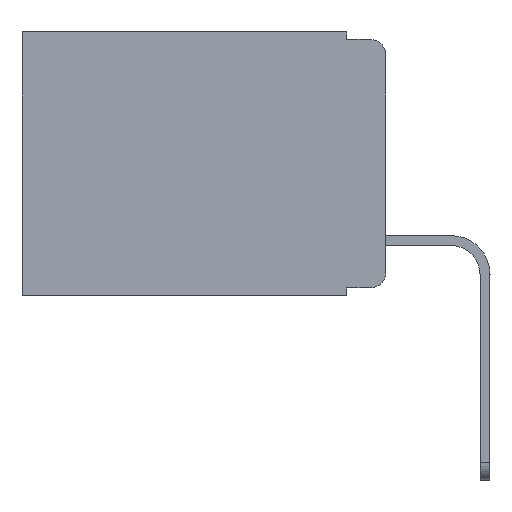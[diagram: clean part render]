
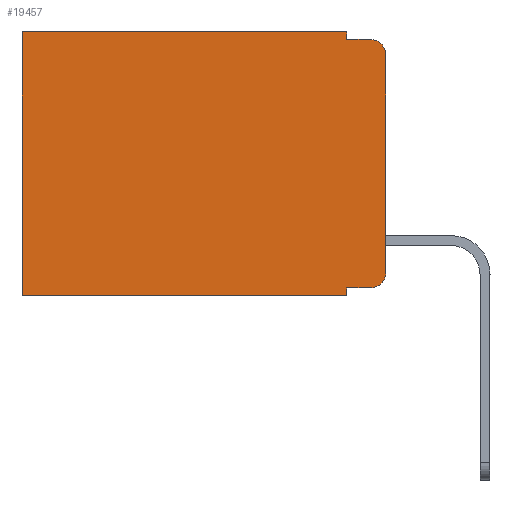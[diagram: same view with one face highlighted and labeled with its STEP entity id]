
A CAD part, left-side view. The second image highlights one B-rep face of the part: STEP entity #19457.
In plain terms, the highlighted planar face has unit normal (-1, 0, 0).
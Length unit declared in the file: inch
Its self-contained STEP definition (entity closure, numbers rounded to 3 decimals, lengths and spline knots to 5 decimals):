
#99 = LINE ( 'NONE', #16720, #21106 ) ;
#116 = VERTEX_POINT ( 'NONE', #7004 ) ;
#700 = CARTESIAN_POINT ( 'NONE',  ( 0.298, 0., 0. ) ) ;
#805 = CARTESIAN_POINT ( 'NONE',  ( 0.298, 0.051, 0. ) ) ;
#884 = EDGE_CURVE ( 'NONE', #15187, #2984, #10639, .T. ) ;
#1410 = CARTESIAN_POINT ( 'NONE',  ( 0.298, 0.02, -0.333 ) ) ;
#1957 = CARTESIAN_POINT ( 'NONE',  ( 0.298, 0.051, -0.343 ) ) ;
#1967 = CARTESIAN_POINT ( 'NONE',  ( 0.298, 0., 0. ) ) ;
#2198 = CIRCLE ( 'NONE', #17597, 0.02 ) ;
#2984 = VERTEX_POINT ( 'NONE', #6720 ) ;
#3014 = ORIENTED_EDGE ( 'NONE', *, *, #12212, .T. ) ;
#3509 = DIRECTION ( 'NONE',  ( 0., -1., 0. ) ) ;
#4703 = CARTESIAN_POINT ( 'NONE',  ( 0.298, 0.473, 0. ) ) ;
#4717 = VERTEX_POINT ( 'NONE', #5454 ) ;
#4890 = LINE ( 'NONE', #700, #11181 ) ;
#5038 = PLANE ( 'NONE',  #6435 ) ;
#5395 = CIRCLE ( 'NONE', #13631, 0.02 ) ;
#5454 = CARTESIAN_POINT ( 'NONE',  ( 0.298, 0.051, 0. ) ) ;
#5501 = DIRECTION ( 'NONE',  ( 0., 0., -1. ) ) ;
#6351 = DIRECTION ( 'NONE',  ( 0., -1., 0. ) ) ;
#6385 = VECTOR ( 'NONE', #14588, 39.37008 ) ;
#6435 = AXIS2_PLACEMENT_3D ( 'NONE', #1967, #9083, #5501 ) ;
#6720 = CARTESIAN_POINT ( 'NONE',  ( 0.298, 0.473, -0.343 ) ) ;
#6921 = VERTEX_POINT ( 'NONE', #4703 ) ;
#6959 = CARTESIAN_POINT ( 'NONE',  ( 0.298, 0.051, -0.01 ) ) ;
#7004 = CARTESIAN_POINT ( 'NONE',  ( 0.298, 0., -0.313 ) ) ;
#7032 = ORIENTED_EDGE ( 'NONE', *, *, #16856, .F. ) ;
#7314 = VERTEX_POINT ( 'NONE', #1410 ) ;
#7860 = DIRECTION ( 'NONE',  ( 0., 0., -1. ) ) ;
#7877 = ORIENTED_EDGE ( 'NONE', *, *, #11622, .T. ) ;
#7976 = VECTOR ( 'NONE', #8120, 39.37008 ) ;
#8120 = DIRECTION ( 'NONE',  ( 0., 0., -1. ) ) ;
#9007 = CARTESIAN_POINT ( 'NONE',  ( 0.298, 0., 0. ) ) ;
#9083 = DIRECTION ( 'NONE',  ( 1., 0., 0. ) ) ;
#9539 = VECTOR ( 'NONE', #22508, 39.37008 ) ;
#9579 = ORIENTED_EDGE ( 'NONE', *, *, #17667, .T. ) ;
#9750 = CARTESIAN_POINT ( 'NONE',  ( 0.298, 0., -0.03 ) ) ;
#9938 = ORIENTED_EDGE ( 'NONE', *, *, #18809, .F. ) ;
#10188 = VERTEX_POINT ( 'NONE', #19893 ) ;
#10415 = VECTOR ( 'NONE', #17415, 39.37008 ) ;
#10639 = LINE ( 'NONE', #13687, #9539 ) ;
#10752 = VERTEX_POINT ( 'NONE', #12371 ) ;
#11143 = ORIENTED_EDGE ( 'NONE', *, *, #15309, .F. ) ;
#11181 = VECTOR ( 'NONE', #12824, 39.37008 ) ;
#11230 = CARTESIAN_POINT ( 'NONE',  ( 0.298, 0.02, -0.313 ) ) ;
#11377 = EDGE_LOOP ( 'NONE', ( #7032, #15712, #9938, #17864, #9579, #7877, #16449, #11143, #3014, #19905 ) ) ;
#11622 = EDGE_CURVE ( 'NONE', #6921, #2984, #13691, .T. ) ;
#12212 = EDGE_CURVE ( 'NONE', #10752, #7314, #99, .T. ) ;
#12371 = CARTESIAN_POINT ( 'NONE',  ( 0.298, 0.051, -0.333 ) ) ;
#12532 = DIRECTION ( 'NONE',  ( -1., 0., 0. ) ) ;
#12554 = DIRECTION ( 'NONE',  ( 0., 0., -1. ) ) ;
#12738 = EDGE_CURVE ( 'NONE', #15353, #19246, #5395, .T. ) ;
#12824 = DIRECTION ( 'NONE',  ( 0., 1., 0. ) ) ;
#13631 = AXIS2_PLACEMENT_3D ( 'NONE', #17773, #12532, #21265 ) ;
#13687 = CARTESIAN_POINT ( 'NONE',  ( 0.298, 0., -0.343 ) ) ;
#13691 = LINE ( 'NONE', #15107, #7976 ) ;
#14102 = VECTOR ( 'NONE', #3509, 39.37008 ) ;
#14457 = FACE_OUTER_BOUND ( 'NONE', #11377, .T. ) ;
#14588 = DIRECTION ( 'NONE',  ( 0., 0., -1. ) ) ;
#15107 = CARTESIAN_POINT ( 'NONE',  ( 0.298, 0.473, 0. ) ) ;
#15187 = VERTEX_POINT ( 'NONE', #1957 ) ;
#15280 = VECTOR ( 'NONE', #12554, 39.37008 ) ;
#15309 = EDGE_CURVE ( 'NONE', #10752, #15187, #21674, .T. ) ;
#15353 = VERTEX_POINT ( 'NONE', #9750 ) ;
#15712 = ORIENTED_EDGE ( 'NONE', *, *, #12738, .T. ) ;
#16305 = LINE ( 'NONE', #6959, #14102 ) ;
#16390 = LINE ( 'NONE', #9007, #15280 ) ;
#16449 = ORIENTED_EDGE ( 'NONE', *, *, #884, .F. ) ;
#16716 = DIRECTION ( 'NONE',  ( -1., 0., 0. ) ) ;
#16720 = CARTESIAN_POINT ( 'NONE',  ( 0.298, 0.051, -0.333 ) ) ;
#16856 = EDGE_CURVE ( 'NONE', #15353, #116, #16390, .T. ) ;
#17415 = DIRECTION ( 'NONE',  ( 0., 0., -1. ) ) ;
#17597 = AXIS2_PLACEMENT_3D ( 'NONE', #11230, #16716, #7860 ) ;
#17667 = EDGE_CURVE ( 'NONE', #4717, #6921, #4890, .T. ) ;
#17773 = CARTESIAN_POINT ( 'NONE',  ( 0.298, 0.02, -0.03 ) ) ;
#17864 = ORIENTED_EDGE ( 'NONE', *, *, #22107, .F. ) ;
#18809 = EDGE_CURVE ( 'NONE', #10188, #19246, #16305, .T. ) ;
#19089 = EDGE_CURVE ( 'NONE', #7314, #116, #2198, .T. ) ;
#19176 = CARTESIAN_POINT ( 'NONE',  ( 0.298, 0.051, 0. ) ) ;
#19246 = VERTEX_POINT ( 'NONE', #22372 ) ;
#19417 = LINE ( 'NONE', #19176, #10415 ) ;
#19457 = ADVANCED_FACE ( 'NONE', ( #14457 ), #5038, .F. ) ;
#19893 = CARTESIAN_POINT ( 'NONE',  ( 0.298, 0.051, -0.01 ) ) ;
#19905 = ORIENTED_EDGE ( 'NONE', *, *, #19089, .T. ) ;
#21106 = VECTOR ( 'NONE', #6351, 39.37008 ) ;
#21265 = DIRECTION ( 'NONE',  ( 0., 0., -1. ) ) ;
#21674 = LINE ( 'NONE', #805, #6385 ) ;
#22107 = EDGE_CURVE ( 'NONE', #4717, #10188, #19417, .T. ) ;
#22372 = CARTESIAN_POINT ( 'NONE',  ( 0.298, 0.02, -0.01 ) ) ;
#22508 = DIRECTION ( 'NONE',  ( 0., 1., 0. ) ) ;
